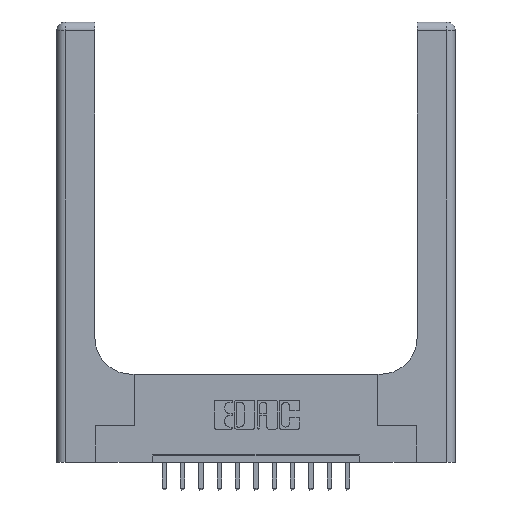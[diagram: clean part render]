
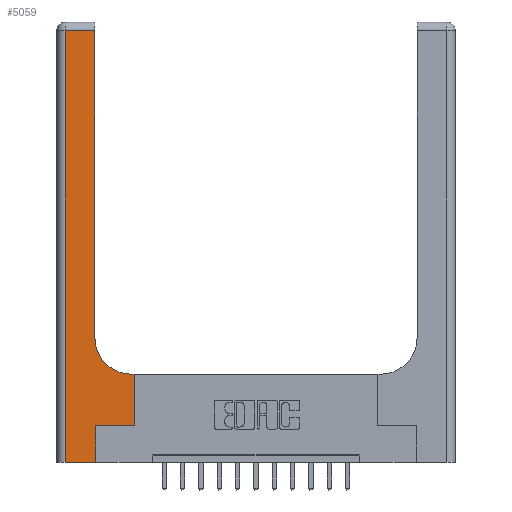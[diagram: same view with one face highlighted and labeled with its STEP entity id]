
A CAD part, top view. The second image highlights one B-rep face of the part: STEP entity #5059.
In plain terms, the highlighted planar face has unit normal (0, 0, 1).
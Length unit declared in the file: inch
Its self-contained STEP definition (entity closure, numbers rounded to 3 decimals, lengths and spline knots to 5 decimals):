
#163 = EDGE_CURVE ( 'NONE', #6158, #12809, #15239, .T. ) ;
#309 = VECTOR ( 'NONE', #6081, 39.37008 ) ;
#425 = ORIENTED_EDGE ( 'NONE', *, *, #14149, .T. ) ;
#536 = VECTOR ( 'NONE', #4107, 39.37008 ) ;
#677 = CARTESIAN_POINT ( 'NONE',  ( 0.51, 0.85, 0.37 ) ) ;
#737 = ORIENTED_EDGE ( 'NONE', *, *, #8182, .T. ) ;
#931 = ORIENTED_EDGE ( 'NONE', *, *, #2901, .T. ) ;
#940 = CARTESIAN_POINT ( 'NONE',  ( 0.06, 0., 0.37 ) ) ;
#1086 = CIRCLE ( 'NONE', #6784, 0.25 ) ;
#1156 = LINE ( 'NONE', #11678, #14119 ) ;
#1372 = CARTESIAN_POINT ( 'NONE',  ( 0.06, 2.94, 0.37 ) ) ;
#1454 = CARTESIAN_POINT ( 'NONE',  ( 0.528, 0.6, 0.37 ) ) ;
#1512 = ORIENTED_EDGE ( 'NONE', *, *, #13016, .T. ) ;
#1656 = CARTESIAN_POINT ( 'NONE',  ( 0.51, 0.6, 0.37 ) ) ;
#1738 = AXIS2_PLACEMENT_3D ( 'NONE', #16039, #14691, #2185 ) ;
#2185 = DIRECTION ( 'NONE',  ( -1., 0., 0. ) ) ;
#2901 = EDGE_CURVE ( 'NONE', #10804, #15229, #6924, .T. ) ;
#2908 = CARTESIAN_POINT ( 'NONE',  ( 0.265, 0.25, 0.37 ) ) ;
#4107 = DIRECTION ( 'NONE',  ( 0., 1., 0. ) ) ;
#4175 = ORIENTED_EDGE ( 'NONE', *, *, #5275, .T. ) ;
#4360 = ORIENTED_EDGE ( 'NONE', *, *, #10310, .T. ) ;
#4796 = CARTESIAN_POINT ( 'NONE',  ( 0.26, 2.94, 0.37 ) ) ;
#5059 = ADVANCED_FACE ( 'NONE', ( #12262 ), #9796, .F. ) ;
#5171 = CARTESIAN_POINT ( 'NONE',  ( 0., 2.94, 0.37 ) ) ;
#5198 = DIRECTION ( 'NONE',  ( 0., 1., 0. ) ) ;
#5275 = EDGE_CURVE ( 'NONE', #12809, #10804, #8160, .T. ) ;
#5301 = VECTOR ( 'NONE', #9012, 39.37008 ) ;
#5657 = LINE ( 'NONE', #11167, #11145 ) ;
#5791 = LINE ( 'NONE', #12439, #14818 ) ;
#6081 = DIRECTION ( 'NONE',  ( 1., 0., 0. ) ) ;
#6158 = VERTEX_POINT ( 'NONE', #10880 ) ;
#6338 = DIRECTION ( 'NONE',  ( 1., 0., 0. ) ) ;
#6618 = CARTESIAN_POINT ( 'NONE',  ( 0.265, 0., 0.37 ) ) ;
#6784 = AXIS2_PLACEMENT_3D ( 'NONE', #677, #14491, #14549 ) ;
#6793 = CARTESIAN_POINT ( 'NONE',  ( 0.265, 0., 0.37 ) ) ;
#6924 = LINE ( 'NONE', #8223, #14745 ) ;
#7049 = ORIENTED_EDGE ( 'NONE', *, *, #14292, .T. ) ;
#7086 = CARTESIAN_POINT ( 'NONE',  ( 0.265, 0.25, 0.37 ) ) ;
#7701 = EDGE_CURVE ( 'NONE', #10205, #10711, #14319, .T. ) ;
#7871 = CARTESIAN_POINT ( 'NONE',  ( 0.26, 3., 0.37 ) ) ;
#8160 = LINE ( 'NONE', #5171, #11474 ) ;
#8182 = EDGE_CURVE ( 'NONE', #11311, #13276, #1156, .T. ) ;
#8223 = CARTESIAN_POINT ( 'NONE',  ( 0.06, 3., 0.37 ) ) ;
#9012 = DIRECTION ( 'NONE',  ( 0., 1., 0. ) ) ;
#9357 = EDGE_LOOP ( 'NONE', ( #12520, #4175, #931, #1512, #15601, #425, #7049, #737, #4360 ) ) ;
#9796 = PLANE ( 'NONE',  #1738 ) ;
#10205 = VERTEX_POINT ( 'NONE', #6793 ) ;
#10310 = EDGE_CURVE ( 'NONE', #13276, #6158, #1086, .T. ) ;
#10711 = VERTEX_POINT ( 'NONE', #2908 ) ;
#10804 = VERTEX_POINT ( 'NONE', #1372 ) ;
#10880 = CARTESIAN_POINT ( 'NONE',  ( 0.26, 0.85, 0.37 ) ) ;
#11145 = VECTOR ( 'NONE', #6338, 39.37008 ) ;
#11167 = CARTESIAN_POINT ( 'NONE',  ( 0., 0., 0.37 ) ) ;
#11311 = VERTEX_POINT ( 'NONE', #1454 ) ;
#11474 = VECTOR ( 'NONE', #13833, 39.37008 ) ;
#11678 = CARTESIAN_POINT ( 'NONE',  ( 0.26, 0.6, 0.37 ) ) ;
#11829 = VERTEX_POINT ( 'NONE', #15141 ) ;
#11979 = DIRECTION ( 'NONE',  ( 0., -1., 0. ) ) ;
#12083 = LINE ( 'NONE', #7086, #309 ) ;
#12262 = FACE_OUTER_BOUND ( 'NONE', #9357, .T. ) ;
#12439 = CARTESIAN_POINT ( 'NONE',  ( 0.528, 0.25, 0.37 ) ) ;
#12520 = ORIENTED_EDGE ( 'NONE', *, *, #163, .T. ) ;
#12809 = VERTEX_POINT ( 'NONE', #4796 ) ;
#13016 = EDGE_CURVE ( 'NONE', #15229, #10205, #5657, .T. ) ;
#13276 = VERTEX_POINT ( 'NONE', #1656 ) ;
#13833 = DIRECTION ( 'NONE',  ( -1., 0., 0. ) ) ;
#14119 = VECTOR ( 'NONE', #14186, 39.37008 ) ;
#14149 = EDGE_CURVE ( 'NONE', #10711, #11829, #12083, .T. ) ;
#14186 = DIRECTION ( 'NONE',  ( -1., 0., 0. ) ) ;
#14292 = EDGE_CURVE ( 'NONE', #11829, #11311, #5791, .T. ) ;
#14319 = LINE ( 'NONE', #6618, #5301 ) ;
#14491 = DIRECTION ( 'NONE',  ( 0., 0., -1. ) ) ;
#14549 = DIRECTION ( 'NONE',  ( 1., 0., 0. ) ) ;
#14691 = DIRECTION ( 'NONE',  ( 0., 0., -1. ) ) ;
#14745 = VECTOR ( 'NONE', #11979, 39.37008 ) ;
#14818 = VECTOR ( 'NONE', #5198, 39.37008 ) ;
#15141 = CARTESIAN_POINT ( 'NONE',  ( 0.528, 0.25, 0.37 ) ) ;
#15229 = VERTEX_POINT ( 'NONE', #940 ) ;
#15239 = LINE ( 'NONE', #7871, #536 ) ;
#15601 = ORIENTED_EDGE ( 'NONE', *, *, #7701, .T. ) ;
#16039 = CARTESIAN_POINT ( 'NONE',  ( 0., 3., 0.37 ) ) ;
